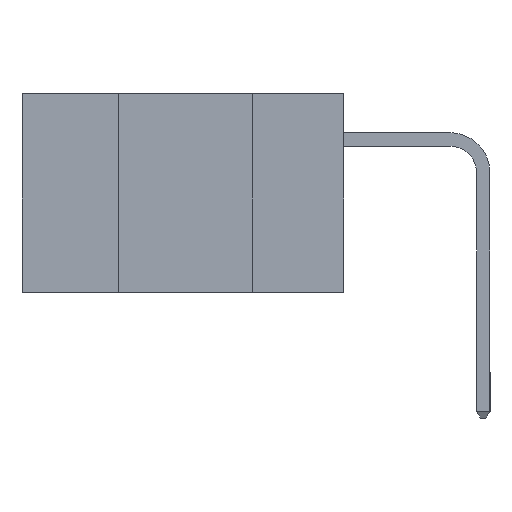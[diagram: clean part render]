
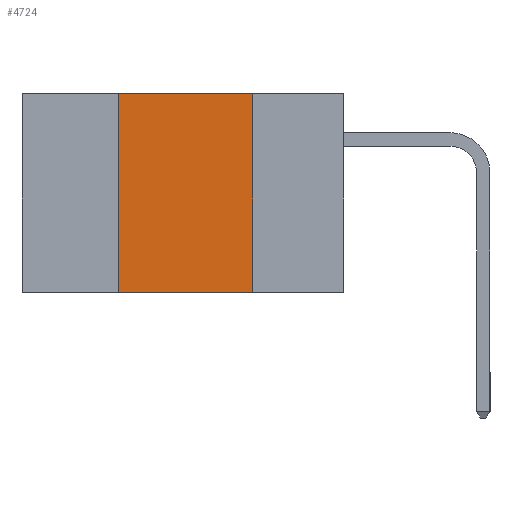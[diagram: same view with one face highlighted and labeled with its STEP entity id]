
A CAD part, left-side view. The second image highlights one B-rep face of the part: STEP entity #4724.
In plain terms, the highlighted planar face has unit normal (-1, 0, 0).
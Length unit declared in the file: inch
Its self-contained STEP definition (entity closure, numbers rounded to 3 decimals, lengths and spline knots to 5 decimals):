
#280 = AXIS2_PLACEMENT_3D ( 'NONE', #870, #2704, #1086 ) ;
#870 = CARTESIAN_POINT ( 'NONE',  ( 0., 0.6, 0. ) ) ;
#1086 = DIRECTION ( 'NONE',  ( 0., 0., -1. ) ) ;
#1149 = CARTESIAN_POINT ( 'NONE',  ( 0., 0.42, 0. ) ) ;
#2704 = DIRECTION ( 'NONE',  ( 1., 0., 0. ) ) ;
#3357 = FACE_OUTER_BOUND ( 'NONE', #3555, .T. ) ;
#3555 = EDGE_LOOP ( 'NONE', ( #12669, #21327, #7333, #14121 ) ) ;
#3575 = CARTESIAN_POINT ( 'NONE',  ( 0., 0.17, 0. ) ) ;
#4160 = DIRECTION ( 'NONE',  ( 0., 0., -1. ) ) ;
#4581 = VERTEX_POINT ( 'NONE', #1149 ) ;
#4724 = ADVANCED_FACE ( 'NONE', ( #3357 ), #9429, .F. ) ;
#5036 = EDGE_CURVE ( 'NONE', #10706, #4581, #22632, .T. ) ;
#5162 = EDGE_CURVE ( 'NONE', #11292, #9015, #16534, .T. ) ;
#5294 = CARTESIAN_POINT ( 'NONE',  ( 0., 0.6, -0.37 ) ) ;
#6299 = DIRECTION ( 'NONE',  ( 0., -1., 0. ) ) ;
#7333 = ORIENTED_EDGE ( 'NONE', *, *, #5036, .F. ) ;
#8130 = CARTESIAN_POINT ( 'NONE',  ( 0., 0.42, -0.37 ) ) ;
#8935 = DIRECTION ( 'NONE',  ( 0., 0., 1. ) ) ;
#9015 = VERTEX_POINT ( 'NONE', #11394 ) ;
#9138 = VECTOR ( 'NONE', #8935, 39.37008 ) ;
#9429 = PLANE ( 'NONE',  #280 ) ;
#9937 = EDGE_CURVE ( 'NONE', #10706, #9015, #14033, .T. ) ;
#10050 = LINE ( 'NONE', #20296, #18032 ) ;
#10706 = VERTEX_POINT ( 'NONE', #8130 ) ;
#11292 = VERTEX_POINT ( 'NONE', #3575 ) ;
#11394 = CARTESIAN_POINT ( 'NONE',  ( 0., 0.17, -0.37 ) ) ;
#12390 = VECTOR ( 'NONE', #15929, 39.37008 ) ;
#12669 = ORIENTED_EDGE ( 'NONE', *, *, #5162, .F. ) ;
#14033 = LINE ( 'NONE', #5294, #12390 ) ;
#14121 = ORIENTED_EDGE ( 'NONE', *, *, #9937, .T. ) ;
#14510 = EDGE_CURVE ( 'NONE', #4581, #11292, #10050, .T. ) ;
#15929 = DIRECTION ( 'NONE',  ( 0., -1., 0. ) ) ;
#16534 = LINE ( 'NONE', #19823, #19560 ) ;
#17923 = CARTESIAN_POINT ( 'NONE',  ( 0., 0.42, 0. ) ) ;
#18032 = VECTOR ( 'NONE', #6299, 39.37008 ) ;
#19560 = VECTOR ( 'NONE', #4160, 39.37008 ) ;
#19823 = CARTESIAN_POINT ( 'NONE',  ( 0., 0.17, 0. ) ) ;
#20296 = CARTESIAN_POINT ( 'NONE',  ( 0., 0.6, 0. ) ) ;
#21327 = ORIENTED_EDGE ( 'NONE', *, *, #14510, .F. ) ;
#22632 = LINE ( 'NONE', #17923, #9138 ) ;
